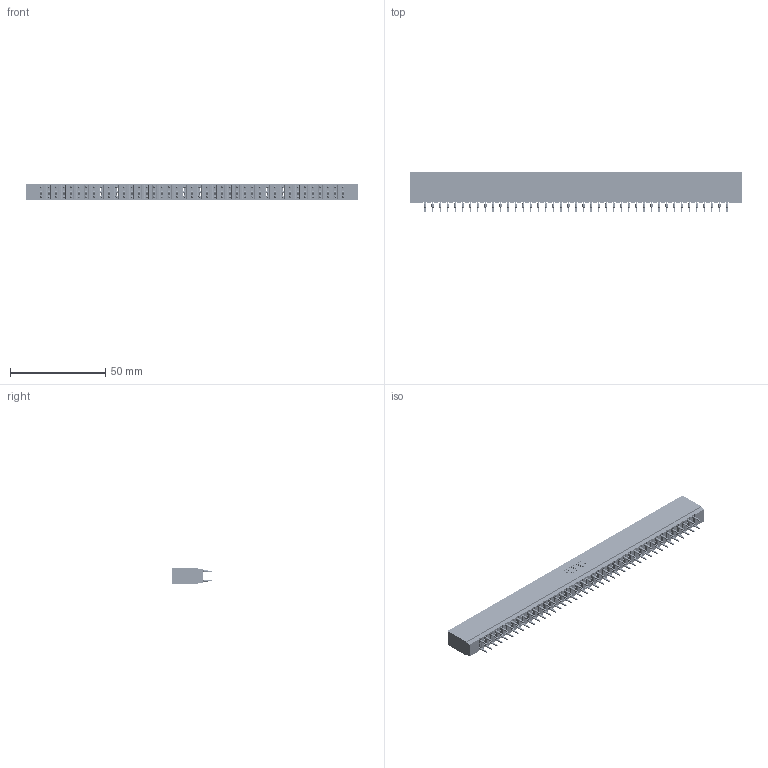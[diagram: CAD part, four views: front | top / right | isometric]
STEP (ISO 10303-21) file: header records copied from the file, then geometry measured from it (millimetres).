
FILE_DESCRIPTION (( 'STEP AP203' ), '1' );
FILE_NAME ('737-082-560-201.STEP', '2020-09-11T08:50:01', ( '' ), ( '' ), 'SwSTEP 2.0', 'SolidWorks 2020', '' );
FILE_SCHEMA (( 'CONFIG_CONTROL_DESIGN' ));
Length unit declared in the file: inch
Products named in the file (3): 737-082-560-201; 745-292-001_560; 737 Part_Insulator Option - 01
Assembly tree (83 placements, depth 2):
  737-082-560-201
    737 Part_Insulator Option - 01
    745-292-001_560  x82
Bounding box: 174.29 x 21.22 x 8.89 mm (x, y, z)
Volume: 17536.5 mm3; surface area: 26923.7 mm2
Topology: 83 solids, 83 shells, 8212 faces, 22477 edges, 14274 vertices
Faces by surface type: plane 4277, cylinder 1803, bspline 1640, torus 492
Entity records: 70810 total; most frequent: CARTESIAN_POINT 12797, ORIENTED_EDGE 12230, DIRECTION 10679, EDGE_CURVE 6115, VECTOR 5679, LINE 5679, VERTEX_POINT 3906, AXIS2_PLACEMENT_3D 2500
